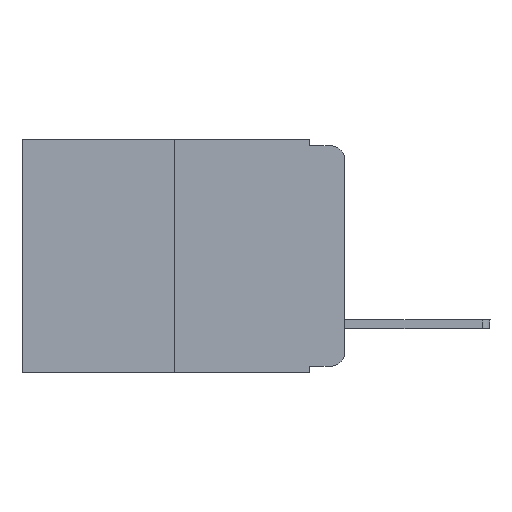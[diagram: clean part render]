
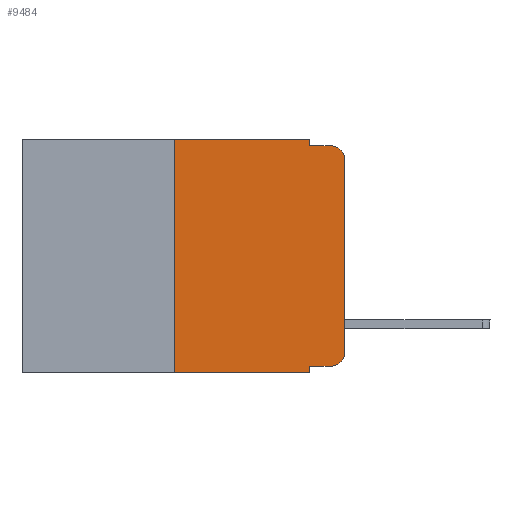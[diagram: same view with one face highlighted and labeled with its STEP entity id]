
A CAD part, left-side view. The second image highlights one B-rep face of the part: STEP entity #9484.
In plain terms, the highlighted planar face has unit normal (-1, 0, 0).
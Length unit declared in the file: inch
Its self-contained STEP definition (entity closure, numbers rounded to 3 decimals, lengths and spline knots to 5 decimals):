
#1240 = DIRECTION ( 'NONE',  ( 0., 0., -1. ) ) ;
#1543 = ORIENTED_EDGE ( 'NONE', *, *, #20240, .F. ) ;
#1796 = CARTESIAN_POINT ( 'NONE',  ( 0., 0.051, 0. ) ) ;
#2096 = DIRECTION ( 'NONE',  ( 0., -1., 0. ) ) ;
#2595 = ORIENTED_EDGE ( 'NONE', *, *, #11912, .T. ) ;
#2899 = LINE ( 'NONE', #11642, #3614 ) ;
#3614 = VECTOR ( 'NONE', #13585, 39.37008 ) ;
#3650 = ORIENTED_EDGE ( 'NONE', *, *, #19835, .F. ) ;
#3701 = EDGE_CURVE ( 'NONE', #20198, #15288, #5326, .T. ) ;
#4169 = DIRECTION ( 'NONE',  ( 0., 0., 1. ) ) ;
#4389 = DIRECTION ( 'NONE',  ( -1., 0., 0. ) ) ;
#5221 = VERTEX_POINT ( 'NONE', #12425 ) ;
#5326 = LINE ( 'NONE', #17637, #7344 ) ;
#5332 = AXIS2_PLACEMENT_3D ( 'NONE', #17656, #7191, #14202 ) ;
#5400 = LINE ( 'NONE', #15873, #7875 ) ;
#5553 = DIRECTION ( 'NONE',  ( 0., -1., 0. ) ) ;
#6020 = VECTOR ( 'NONE', #15899, 39.37008 ) ;
#6324 = CARTESIAN_POINT ( 'NONE',  ( 0., 0.25, -0.343 ) ) ;
#6636 = VERTEX_POINT ( 'NONE', #7281 ) ;
#6786 = CIRCLE ( 'NONE', #5332, 0.02 ) ;
#7191 = DIRECTION ( 'NONE',  ( -1., 0., 0. ) ) ;
#7281 = CARTESIAN_POINT ( 'NONE',  ( 0., 0.051, -0.333 ) ) ;
#7344 = VECTOR ( 'NONE', #21324, 39.37008 ) ;
#7386 = EDGE_CURVE ( 'NONE', #6636, #15288, #10536, .T. ) ;
#7438 = CARTESIAN_POINT ( 'NONE',  ( 0., 0.051, -0.01 ) ) ;
#7494 = VECTOR ( 'NONE', #5553, 39.37008 ) ;
#7518 = VECTOR ( 'NONE', #17309, 39.37008 ) ;
#7620 = CARTESIAN_POINT ( 'NONE',  ( 0., 0.02, -0.03 ) ) ;
#7875 = VECTOR ( 'NONE', #8976, 39.37008 ) ;
#7961 = VERTEX_POINT ( 'NONE', #21208 ) ;
#7984 = EDGE_CURVE ( 'NONE', #6636, #19858, #9008, .T. ) ;
#8256 = ORIENTED_EDGE ( 'NONE', *, *, #7386, .F. ) ;
#8311 = ORIENTED_EDGE ( 'NONE', *, *, #13808, .F. ) ;
#8347 = AXIS2_PLACEMENT_3D ( 'NONE', #7620, #4389, #14619 ) ;
#8653 = ORIENTED_EDGE ( 'NONE', *, *, #7984, .T. ) ;
#8907 = CARTESIAN_POINT ( 'NONE',  ( 0., 0.25, 0. ) ) ;
#8976 = DIRECTION ( 'NONE',  ( 0., 0., 1. ) ) ;
#9008 = LINE ( 'NONE', #19483, #19622 ) ;
#9233 = CARTESIAN_POINT ( 'NONE',  ( 0., 0., 0. ) ) ;
#9484 = ADVANCED_FACE ( 'NONE', ( #17240 ), #19081, .F. ) ;
#10359 = ORIENTED_EDGE ( 'NONE', *, *, #22379, .T. ) ;
#10536 = LINE ( 'NONE', #1796, #7518 ) ;
#11606 = DIRECTION ( 'NONE',  ( 1., 0., 0. ) ) ;
#11642 = CARTESIAN_POINT ( 'NONE',  ( 0., 0.051, -0.01 ) ) ;
#11912 = EDGE_CURVE ( 'NONE', #5221, #18318, #14735, .T. ) ;
#11994 = ORIENTED_EDGE ( 'NONE', *, *, #20711, .T. ) ;
#12219 = LINE ( 'NONE', #19230, #6020 ) ;
#12425 = CARTESIAN_POINT ( 'NONE',  ( 0., 0., -0.313 ) ) ;
#12903 = CARTESIAN_POINT ( 'NONE',  ( 0., 0., -0.03 ) ) ;
#13192 = CARTESIAN_POINT ( 'NONE',  ( 0., 0.051, 0. ) ) ;
#13585 = DIRECTION ( 'NONE',  ( 0., -1., 0. ) ) ;
#13808 = EDGE_CURVE ( 'NONE', #16243, #7961, #2899, .T. ) ;
#14138 = ORIENTED_EDGE ( 'NONE', *, *, #19435, .F. ) ;
#14202 = DIRECTION ( 'NONE',  ( 0., 0., -1. ) ) ;
#14509 = AXIS2_PLACEMENT_3D ( 'NONE', #20696, #11606, #1240 ) ;
#14619 = DIRECTION ( 'NONE',  ( 0., 0., -1. ) ) ;
#14735 = LINE ( 'NONE', #9233, #17551 ) ;
#15288 = VERTEX_POINT ( 'NONE', #19471 ) ;
#15650 = ORIENTED_EDGE ( 'NONE', *, *, #3701, .T. ) ;
#15873 = CARTESIAN_POINT ( 'NONE',  ( 0., 0.25, 0. ) ) ;
#15899 = DIRECTION ( 'NONE',  ( 0., 0., -1. ) ) ;
#16151 = CARTESIAN_POINT ( 'NONE',  ( 0., 0.473, 0. ) ) ;
#16243 = VERTEX_POINT ( 'NONE', #7438 ) ;
#17240 = FACE_OUTER_BOUND ( 'NONE', #21642, .T. ) ;
#17309 = DIRECTION ( 'NONE',  ( 0., 0., -1. ) ) ;
#17427 = VERTEX_POINT ( 'NONE', #13192 ) ;
#17551 = VECTOR ( 'NONE', #4169, 39.37008 ) ;
#17637 = CARTESIAN_POINT ( 'NONE',  ( 0., 0.473, -0.343 ) ) ;
#17656 = CARTESIAN_POINT ( 'NONE',  ( 0., 0.02, -0.313 ) ) ;
#18109 = VERTEX_POINT ( 'NONE', #8907 ) ;
#18318 = VERTEX_POINT ( 'NONE', #12903 ) ;
#19081 = PLANE ( 'NONE',  #14509 ) ;
#19230 = CARTESIAN_POINT ( 'NONE',  ( 0., 0.051, 0. ) ) ;
#19435 = EDGE_CURVE ( 'NONE', #18109, #17427, #21232, .T. ) ;
#19471 = CARTESIAN_POINT ( 'NONE',  ( 0., 0.051, -0.343 ) ) ;
#19483 = CARTESIAN_POINT ( 'NONE',  ( 0., 0.051, -0.333 ) ) ;
#19622 = VECTOR ( 'NONE', #2096, 39.37008 ) ;
#19835 = EDGE_CURVE ( 'NONE', #17427, #16243, #12219, .T. ) ;
#19858 = VERTEX_POINT ( 'NONE', #21198 ) ;
#20198 = VERTEX_POINT ( 'NONE', #6324 ) ;
#20240 = EDGE_CURVE ( 'NONE', #20198, #18109, #5400, .T. ) ;
#20696 = CARTESIAN_POINT ( 'NONE',  ( 0., 0.473, 0. ) ) ;
#20711 = EDGE_CURVE ( 'NONE', #19858, #5221, #6786, .T. ) ;
#21198 = CARTESIAN_POINT ( 'NONE',  ( 0., 0.02, -0.333 ) ) ;
#21208 = CARTESIAN_POINT ( 'NONE',  ( 0., 0.02, -0.01 ) ) ;
#21232 = LINE ( 'NONE', #16151, #7494 ) ;
#21324 = DIRECTION ( 'NONE',  ( 0., -1., 0. ) ) ;
#21642 = EDGE_LOOP ( 'NONE', ( #2595, #10359, #8311, #3650, #14138, #1543, #15650, #8256, #8653, #11994 ) ) ;
#22328 = CIRCLE ( 'NONE', #8347, 0.02 ) ;
#22379 = EDGE_CURVE ( 'NONE', #18318, #7961, #22328, .T. ) ;
